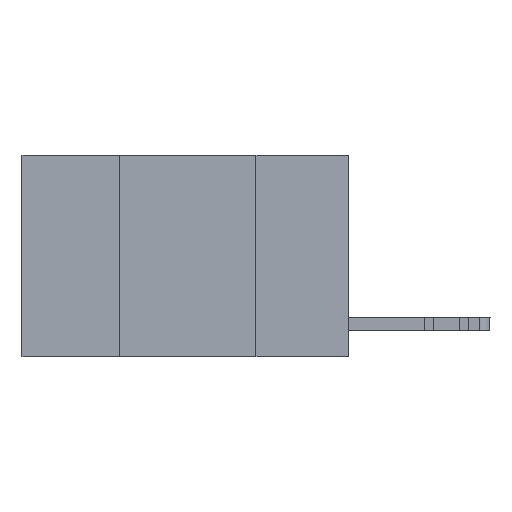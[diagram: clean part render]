
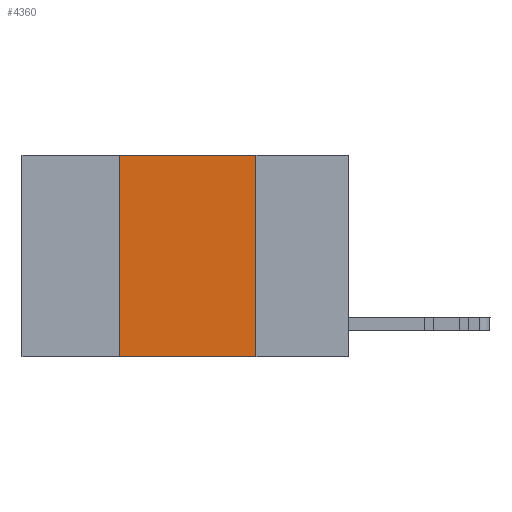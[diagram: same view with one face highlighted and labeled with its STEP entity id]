
A CAD part, left-side view. The second image highlights one B-rep face of the part: STEP entity #4360.
In plain terms, the highlighted planar face has unit normal (-1, 0, 0).
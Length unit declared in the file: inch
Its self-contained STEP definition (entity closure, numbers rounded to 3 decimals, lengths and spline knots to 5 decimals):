
#442 = ORIENTED_EDGE ( 'NONE', *, *, #26107, .F. ) ;
#1155 = DIRECTION ( 'NONE',  ( 0., -1., 0. ) ) ;
#1659 = DIRECTION ( 'NONE',  ( 0., 0., 1. ) ) ;
#1805 = EDGE_CURVE ( 'NONE', #25286, #19969, #23862, .T. ) ;
#1807 = ORIENTED_EDGE ( 'NONE', *, *, #17732, .T. ) ;
#2305 = VECTOR ( 'NONE', #13898, 39.37008 ) ;
#4360 = ADVANCED_FACE ( 'NONE', ( #23293 ), #8935, .F. ) ;
#6583 = VERTEX_POINT ( 'NONE', #10671 ) ;
#6838 = CARTESIAN_POINT ( 'NONE',  ( 0., 0.6, 0. ) ) ;
#8935 = PLANE ( 'NONE',  #26751 ) ;
#9356 = LINE ( 'NONE', #23557, #19707 ) ;
#9663 = CARTESIAN_POINT ( 'NONE',  ( 0., 0.6, 0. ) ) ;
#10638 = EDGE_LOOP ( 'NONE', ( #26288, #16510, #442, #1807 ) ) ;
#10671 = CARTESIAN_POINT ( 'NONE',  ( 0., 0.42, 0. ) ) ;
#11027 = DIRECTION ( 'NONE',  ( 0., 0., -1. ) ) ;
#11112 = DIRECTION ( 'NONE',  ( 0., -1., 0. ) ) ;
#12567 = LINE ( 'NONE', #16267, #22361 ) ;
#13848 = CARTESIAN_POINT ( 'NONE',  ( 0., 0.17, 0. ) ) ;
#13898 = DIRECTION ( 'NONE',  ( 0., 0., -1. ) ) ;
#15052 = DIRECTION ( 'NONE',  ( 1., 0., 0. ) ) ;
#16267 = CARTESIAN_POINT ( 'NONE',  ( 0., 0.42, 0. ) ) ;
#16510 = ORIENTED_EDGE ( 'NONE', *, *, #17921, .F. ) ;
#16588 = CARTESIAN_POINT ( 'NONE',  ( 0., 0.17, -0.37 ) ) ;
#17732 = EDGE_CURVE ( 'NONE', #23808, #19969, #9356, .T. ) ;
#17921 = EDGE_CURVE ( 'NONE', #6583, #25286, #19032, .T. ) ;
#18703 = CARTESIAN_POINT ( 'NONE',  ( 0., 0.42, -0.37 ) ) ;
#19032 = LINE ( 'NONE', #9663, #19678 ) ;
#19678 = VECTOR ( 'NONE', #1155, 39.37008 ) ;
#19707 = VECTOR ( 'NONE', #11112, 39.37008 ) ;
#19969 = VERTEX_POINT ( 'NONE', #16588 ) ;
#21462 = CARTESIAN_POINT ( 'NONE',  ( 0., 0.17, 0. ) ) ;
#22361 = VECTOR ( 'NONE', #1659, 39.37008 ) ;
#23293 = FACE_OUTER_BOUND ( 'NONE', #10638, .T. ) ;
#23557 = CARTESIAN_POINT ( 'NONE',  ( 0., 0.6, -0.37 ) ) ;
#23808 = VERTEX_POINT ( 'NONE', #18703 ) ;
#23862 = LINE ( 'NONE', #13848, #2305 ) ;
#25286 = VERTEX_POINT ( 'NONE', #21462 ) ;
#26107 = EDGE_CURVE ( 'NONE', #23808, #6583, #12567, .T. ) ;
#26288 = ORIENTED_EDGE ( 'NONE', *, *, #1805, .F. ) ;
#26751 = AXIS2_PLACEMENT_3D ( 'NONE', #6838, #15052, #11027 ) ;
